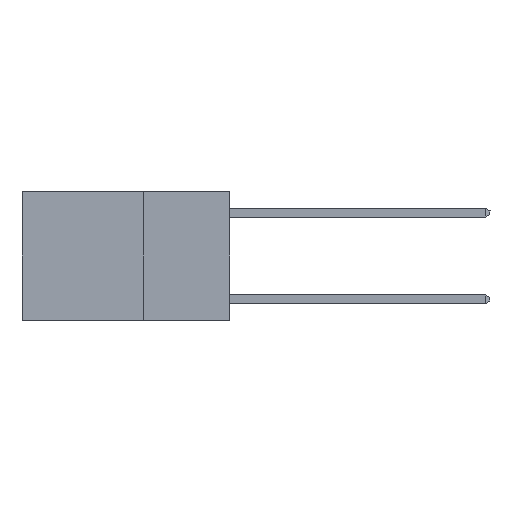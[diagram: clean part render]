
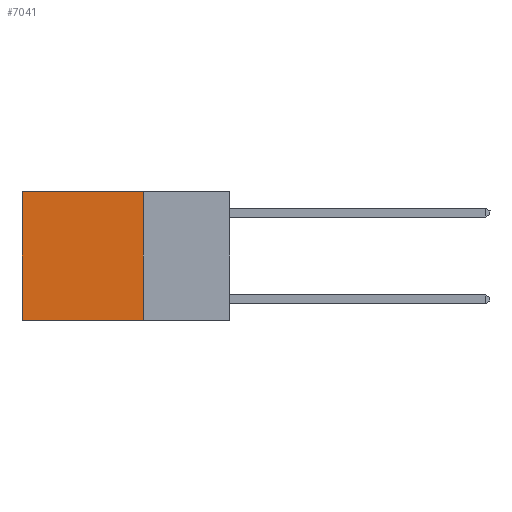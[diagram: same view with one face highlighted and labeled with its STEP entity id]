
A CAD part, left-side view. The second image highlights one B-rep face of the part: STEP entity #7041.
In plain terms, the highlighted planar face has unit normal (-1, 0, 0).
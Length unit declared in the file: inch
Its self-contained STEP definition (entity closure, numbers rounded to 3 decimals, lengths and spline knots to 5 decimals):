
#653 = VERTEX_POINT ( 'NONE', #5588 ) ;
#883 = DIRECTION ( 'NONE',  ( 0., 0., -1. ) ) ;
#1014 = ORIENTED_EDGE ( 'NONE', *, *, #16006, .F. ) ;
#1228 = DIRECTION ( 'NONE',  ( 0., 1., 0. ) ) ;
#1797 = CARTESIAN_POINT ( 'NONE',  ( 0.2625, 0.25, 0. ) ) ;
#2039 = CARTESIAN_POINT ( 'NONE',  ( 0.2625, 0.25, 0. ) ) ;
#2183 = CARTESIAN_POINT ( 'NONE',  ( 0.2625, 0.6, 0. ) ) ;
#3088 = VECTOR ( 'NONE', #1228, 39.37008 ) ;
#3363 = CARTESIAN_POINT ( 'NONE',  ( 0.2625, 0.25, 0. ) ) ;
#3685 = VECTOR ( 'NONE', #6381, 39.37008 ) ;
#4075 = LINE ( 'NONE', #5142, #3685 ) ;
#4501 = ORIENTED_EDGE ( 'NONE', *, *, #14317, .T. ) ;
#4615 = DIRECTION ( 'NONE',  ( 0., 0., -1. ) ) ;
#4618 = PLANE ( 'NONE',  #7776 ) ;
#4737 = VECTOR ( 'NONE', #10903, 39.37008 ) ;
#5142 = CARTESIAN_POINT ( 'NONE',  ( 0.2625, 0.25, 0. ) ) ;
#5588 = CARTESIAN_POINT ( 'NONE',  ( 0.2625, 0.25, -0.37 ) ) ;
#6381 = DIRECTION ( 'NONE',  ( 0., 1., 0. ) ) ;
#6756 = LINE ( 'NONE', #9973, #3088 ) ;
#7041 = ADVANCED_FACE ( 'NONE', ( #7685 ), #4618, .F. ) ;
#7685 = FACE_OUTER_BOUND ( 'NONE', #10661, .T. ) ;
#7776 = AXIS2_PLACEMENT_3D ( 'NONE', #2039, #8364, #883 ) ;
#7847 = CARTESIAN_POINT ( 'NONE',  ( 0.2625, 0.6, 0. ) ) ;
#8026 = LINE ( 'NONE', #2183, #4737 ) ;
#8088 = VERTEX_POINT ( 'NONE', #7847 ) ;
#8364 = DIRECTION ( 'NONE',  ( 1., 0., 0. ) ) ;
#8409 = EDGE_CURVE ( 'NONE', #8088, #14518, #8026, .T. ) ;
#9230 = LINE ( 'NONE', #3363, #15360 ) ;
#9405 = CARTESIAN_POINT ( 'NONE',  ( 0.2625, 0.6, -0.37 ) ) ;
#9973 = CARTESIAN_POINT ( 'NONE',  ( 0.2625, 0.25, -0.37 ) ) ;
#10661 = EDGE_LOOP ( 'NONE', ( #13477, #13286, #1014, #4501 ) ) ;
#10827 = EDGE_CURVE ( 'NONE', #653, #14518, #6756, .T. ) ;
#10903 = DIRECTION ( 'NONE',  ( 0., 0., -1. ) ) ;
#11800 = VERTEX_POINT ( 'NONE', #1797 ) ;
#13286 = ORIENTED_EDGE ( 'NONE', *, *, #10827, .F. ) ;
#13477 = ORIENTED_EDGE ( 'NONE', *, *, #8409, .T. ) ;
#14317 = EDGE_CURVE ( 'NONE', #11800, #8088, #4075, .T. ) ;
#14518 = VERTEX_POINT ( 'NONE', #9405 ) ;
#15360 = VECTOR ( 'NONE', #4615, 39.37008 ) ;
#16006 = EDGE_CURVE ( 'NONE', #11800, #653, #9230, .T. ) ;
